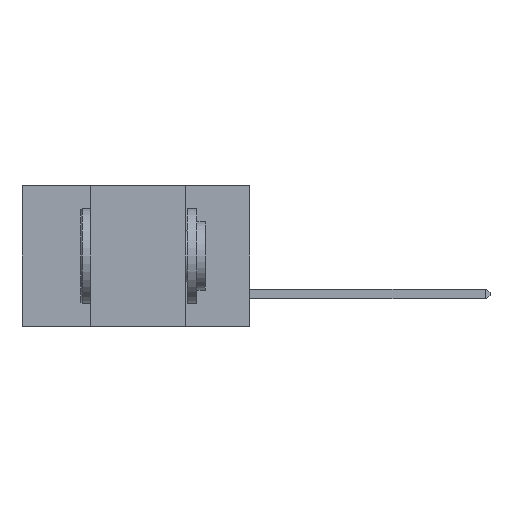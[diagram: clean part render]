
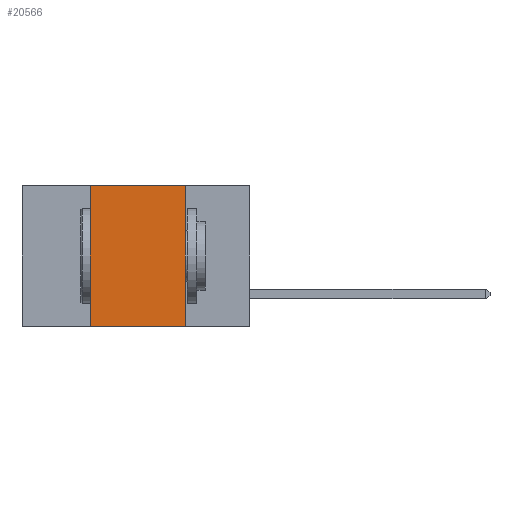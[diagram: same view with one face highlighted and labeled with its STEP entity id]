
A CAD part, left-side view. The second image highlights one B-rep face of the part: STEP entity #20566.
In plain terms, the highlighted planar face has unit normal (-1, 0, 0).
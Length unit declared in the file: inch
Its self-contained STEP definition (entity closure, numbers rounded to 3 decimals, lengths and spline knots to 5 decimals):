
#108 = DIRECTION ( 'NONE',  ( 0., -1., 0. ) ) ;
#560 = CARTESIAN_POINT ( 'NONE',  ( 0., 0.6, 0. ) ) ;
#1229 = CARTESIAN_POINT ( 'NONE',  ( 0., 0.17, 0. ) ) ;
#2053 = ORIENTED_EDGE ( 'NONE', *, *, #14809, .F. ) ;
#3931 = CARTESIAN_POINT ( 'NONE',  ( 0., 0.42, 0. ) ) ;
#4317 = EDGE_LOOP ( 'NONE', ( #2053, #17541, #21448, #28046 ) ) ;
#7292 = EDGE_CURVE ( 'NONE', #12859, #26256, #27964, .T. ) ;
#7703 = LINE ( 'NONE', #31918, #26335 ) ;
#7850 = VECTOR ( 'NONE', #11960, 39.37008 ) ;
#11960 = DIRECTION ( 'NONE',  ( 0., 0., -1. ) ) ;
#12521 = CARTESIAN_POINT ( 'NONE',  ( 0., 0.6, 0. ) ) ;
#12859 = VERTEX_POINT ( 'NONE', #3931 ) ;
#14809 = EDGE_CURVE ( 'NONE', #26256, #19244, #21396, .T. ) ;
#15024 = VECTOR ( 'NONE', #108, 39.37008 ) ;
#15097 = DIRECTION ( 'NONE',  ( 1., 0., 0. ) ) ;
#15373 = CARTESIAN_POINT ( 'NONE',  ( 0., 0.17, 0. ) ) ;
#17541 = ORIENTED_EDGE ( 'NONE', *, *, #7292, .F. ) ;
#18367 = CARTESIAN_POINT ( 'NONE',  ( 0., 0.6, -0.37 ) ) ;
#19244 = VERTEX_POINT ( 'NONE', #19287 ) ;
#19287 = CARTESIAN_POINT ( 'NONE',  ( 0., 0.17, -0.37 ) ) ;
#20566 = ADVANCED_FACE ( 'NONE', ( #28819 ), #27580, .F. ) ;
#21200 = VERTEX_POINT ( 'NONE', #28576 ) ;
#21396 = LINE ( 'NONE', #1229, #7850 ) ;
#21448 = ORIENTED_EDGE ( 'NONE', *, *, #23209, .F. ) ;
#22067 = DIRECTION ( 'NONE',  ( 0., 0., 1. ) ) ;
#23209 = EDGE_CURVE ( 'NONE', #21200, #12859, #7703, .T. ) ;
#23749 = AXIS2_PLACEMENT_3D ( 'NONE', #12521, #15097, #32517 ) ;
#26256 = VERTEX_POINT ( 'NONE', #15373 ) ;
#26335 = VECTOR ( 'NONE', #22067, 39.37008 ) ;
#27233 = VECTOR ( 'NONE', #31241, 39.37008 ) ;
#27580 = PLANE ( 'NONE',  #23749 ) ;
#27964 = LINE ( 'NONE', #560, #27233 ) ;
#28046 = ORIENTED_EDGE ( 'NONE', *, *, #31502, .T. ) ;
#28300 = LINE ( 'NONE', #18367, #15024 ) ;
#28576 = CARTESIAN_POINT ( 'NONE',  ( 0., 0.42, -0.37 ) ) ;
#28819 = FACE_OUTER_BOUND ( 'NONE', #4317, .T. ) ;
#31241 = DIRECTION ( 'NONE',  ( 0., -1., 0. ) ) ;
#31502 = EDGE_CURVE ( 'NONE', #21200, #19244, #28300, .T. ) ;
#31918 = CARTESIAN_POINT ( 'NONE',  ( 0., 0.42, 0. ) ) ;
#32517 = DIRECTION ( 'NONE',  ( 0., 0., -1. ) ) ;
